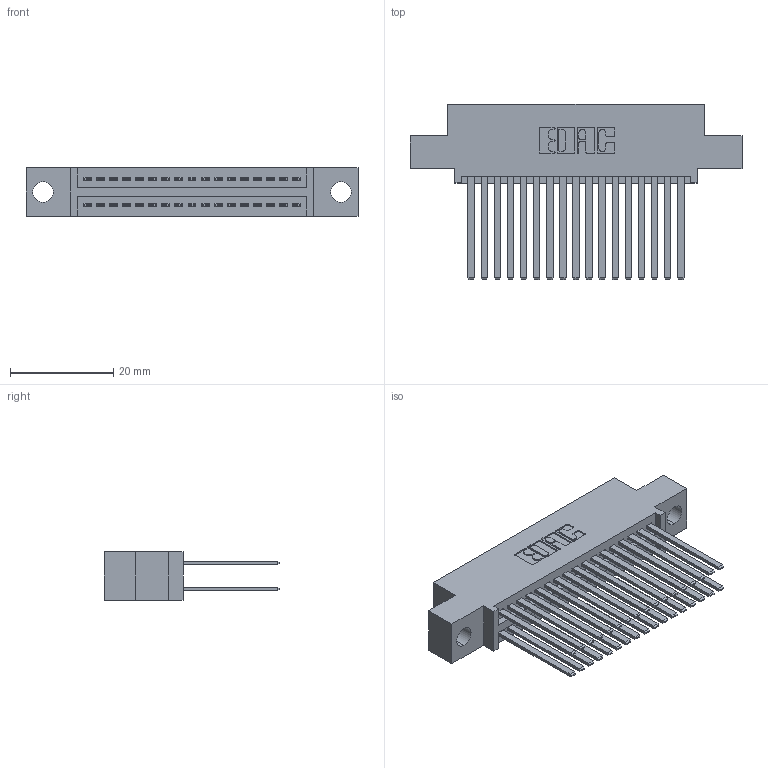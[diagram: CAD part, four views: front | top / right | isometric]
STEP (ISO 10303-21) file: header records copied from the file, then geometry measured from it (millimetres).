
FILE_DESCRIPTION (( 'STEP AP203' ), '1' );
FILE_NAME ('345-034-544-504.STEP', '2021-05-20T00:07:59', ( '' ), ( '' ), 'SwSTEP 2.0', 'SolidWorks 2020', '' );
FILE_SCHEMA (( 'CONFIG_CONTROL_DESIGN' ));
Length unit declared in the file: inch
Products named in the file (3): 345 Part_0.110 Offset - 0.156 Dia-TI; 345-034-544-504; 345-292-001_345-293-144
Assembly tree (35 placements, depth 2):
  345-034-544-504
    345 Part_0.110 Offset - 0.156 Dia-TI
    345-292-001_345-293-144  x34
Bounding box: 64.39 x 33.96 x 9.4 mm (x, y, z)
Volume: 6320.1 mm3; surface area: 10199.3 mm2
Topology: 35 solids, 35 shells, 1640 faces, 4843 edges, 3182 vertices
Faces by surface type: plane 1084, cylinder 556
Entity records: 17071 total; most frequent: CARTESIAN_POINT 2890, ORIENTED_EDGE 2822, DIRECTION 2575, EDGE_CURVE 1411, LINE 1215, VECTOR 1215, VERTEX_POINT 938, AXIS2_PLACEMENT_3D 680
